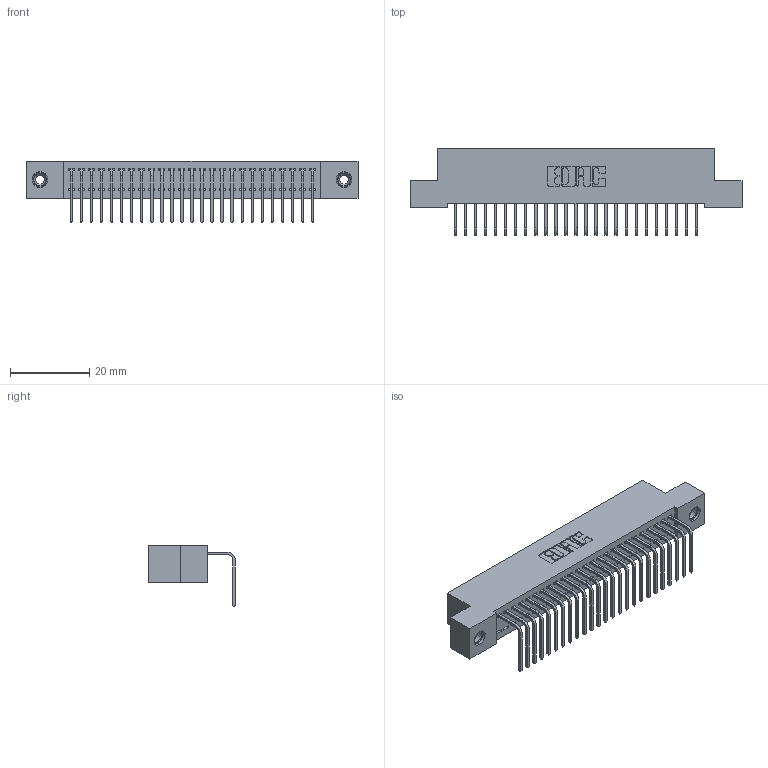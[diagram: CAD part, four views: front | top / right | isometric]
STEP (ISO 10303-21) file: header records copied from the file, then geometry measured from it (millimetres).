
FILE_DESCRIPTION (( 'STEP AP203' ), '1' );
FILE_NAME ('342-025-558-108.STEP', '2019-10-02T00:47:42', ( '' ), ( '' ), 'SwSTEP 2.0', 'SolidWorks 2016', '' );
FILE_SCHEMA (( 'CONFIG_CONTROL_DESIGN' ));
Length unit declared in the file: inch
Products named in the file (4): 345-292-001_558 Tail - 2; 345-250-001_345-250-003-102; 342-025-558-108; 342 Part_TI
Assembly tree (28 placements, depth 2):
  342-025-558-108
    342 Part_TI
    345-292-001_558 Tail - 2  x25
    345-250-001_345-250-003-102  x2
Bounding box: 83.82 x 21.91 x 15.62 mm (x, y, z)
Volume: 7364.3 mm3; surface area: 10987.6 mm2
Topology: 28 solids, 28 shells, 1670 faces, 4985 edges, 3282 vertices
Faces by surface type: plane 1198, cylinder 456, cone 12, torus 4
Entity records: 18620 total; most frequent: CARTESIAN_POINT 3196, ORIENTED_EDGE 3150, DIRECTION 2763, EDGE_CURVE 1575, VECTOR 1427, LINE 1427, VERTEX_POINT 1044, AXIS2_PLACEMENT_3D 668
